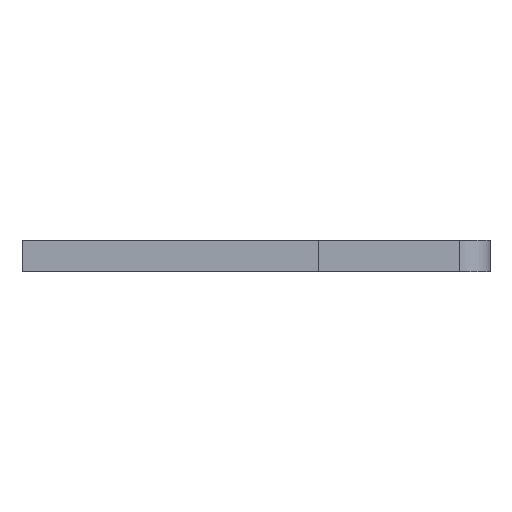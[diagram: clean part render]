
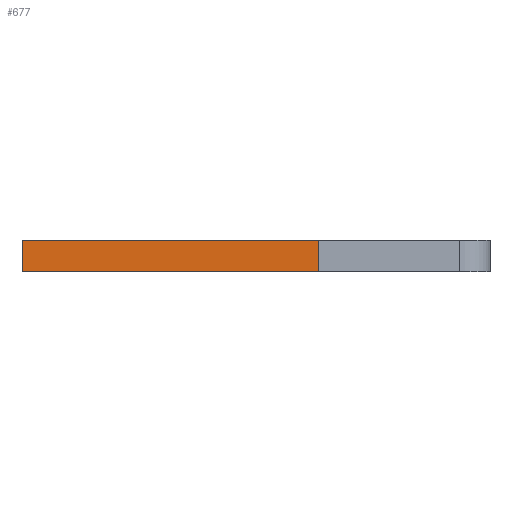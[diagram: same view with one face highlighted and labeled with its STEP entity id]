
A CAD part, left-side view. The second image highlights one B-rep face of the part: STEP entity #677.
In plain terms, the highlighted face is planar.
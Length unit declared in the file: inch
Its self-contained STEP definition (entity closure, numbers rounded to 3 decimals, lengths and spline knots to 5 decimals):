
#5 = EDGE_CURVE ( 'NONE', #920, #891, #407, .T. ) ;
#35 = EDGE_CURVE ( 'NONE', #464, #920, #175, .T. ) ;
#48 = LINE ( 'NONE', #753, #636 ) ;
#54 = ORIENTED_EDGE ( 'NONE', *, *, #721, .T. ) ;
#123 = ORIENTED_EDGE ( 'NONE', *, *, #5, .F. ) ;
#175 = LINE ( 'NONE', #615, #618 ) ;
#183 = CARTESIAN_POINT ( 'NONE',  ( 0.01, 0.15, -0.04 ) ) ;
#191 = DIRECTION ( 'NONE',  ( 0., 1., 0. ) ) ;
#211 = VECTOR ( 'NONE', #333, 39.37008 ) ;
#214 = VECTOR ( 'NONE', #836, 39.37008 ) ;
#252 = CARTESIAN_POINT ( 'NONE',  ( -0.01, 0.15, -0.04 ) ) ;
#264 = CARTESIAN_POINT ( 'NONE',  ( -0.01, 0.15, -0.04 ) ) ;
#326 = DIRECTION ( 'NONE',  ( 0., 0., 1. ) ) ;
#333 = DIRECTION ( 'NONE',  ( 0., 1., 0. ) ) ;
#351 = AXIS2_PLACEMENT_3D ( 'NONE', #183, #326, #397 ) ;
#367 = CARTESIAN_POINT ( 'NONE',  ( -0.01, -0.04, -0.04 ) ) ;
#375 = VERTEX_POINT ( 'NONE', #367 ) ;
#394 = PLANE ( 'NONE',  #351 ) ;
#397 = DIRECTION ( 'NONE',  ( 1., 0., 0. ) ) ;
#401 = CARTESIAN_POINT ( 'NONE',  ( 0.01, 0.15, -0.04 ) ) ;
#407 = LINE ( 'NONE', #401, #214 ) ;
#414 = LINE ( 'NONE', #252, #211 ) ;
#464 = VERTEX_POINT ( 'NONE', #743 ) ;
#478 = CARTESIAN_POINT ( 'NONE',  ( 0.01, 0.15, -0.04 ) ) ;
#515 = EDGE_LOOP ( 'NONE', ( #879, #123, #871, #54 ) ) ;
#615 = CARTESIAN_POINT ( 'NONE',  ( 0.01, 0.15, -0.04 ) ) ;
#618 = VECTOR ( 'NONE', #191, 39.37008 ) ;
#636 = VECTOR ( 'NONE', #674, 39.37008 ) ;
#674 = DIRECTION ( 'NONE',  ( -1., 0., 0. ) ) ;
#677 = ADVANCED_FACE ( 'NONE', ( #856 ), #394, .F. ) ;
#721 = EDGE_CURVE ( 'NONE', #464, #375, #48, .T. ) ;
#743 = CARTESIAN_POINT ( 'NONE',  ( 0.01, -0.04, -0.04 ) ) ;
#753 = CARTESIAN_POINT ( 'NONE',  ( 0.01, -0.04, -0.04 ) ) ;
#831 = EDGE_CURVE ( 'NONE', #375, #891, #414, .T. ) ;
#836 = DIRECTION ( 'NONE',  ( -1., 0., 0. ) ) ;
#856 = FACE_OUTER_BOUND ( 'NONE', #515, .T. ) ;
#871 = ORIENTED_EDGE ( 'NONE', *, *, #35, .F. ) ;
#879 = ORIENTED_EDGE ( 'NONE', *, *, #831, .T. ) ;
#891 = VERTEX_POINT ( 'NONE', #264 ) ;
#920 = VERTEX_POINT ( 'NONE', #478 ) ;
